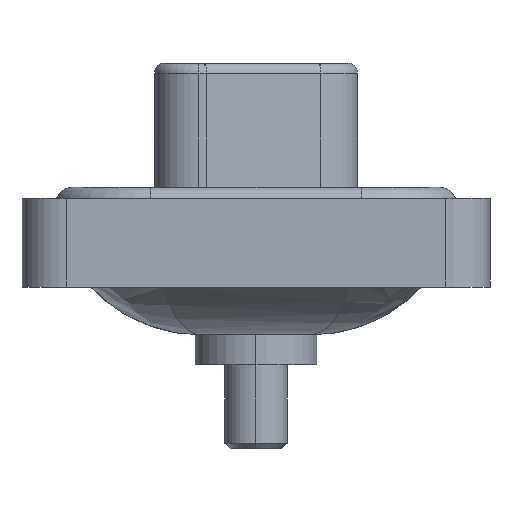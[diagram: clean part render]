
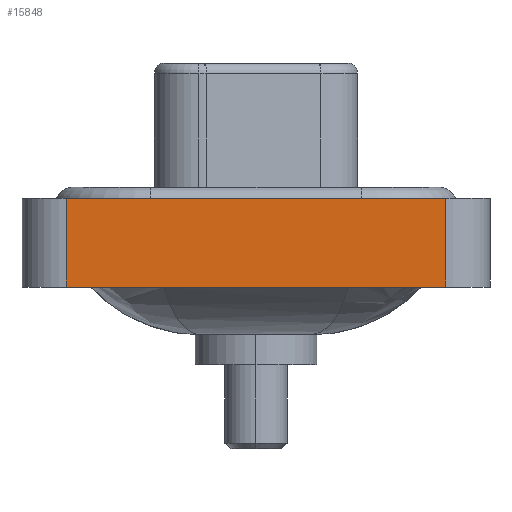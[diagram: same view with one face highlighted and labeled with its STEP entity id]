
A CAD part, left-side view. The second image highlights one B-rep face of the part: STEP entity #15848.
In plain terms, the highlighted planar face has unit normal (-1, 0, 0).
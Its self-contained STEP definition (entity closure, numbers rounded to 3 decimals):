
#290 = DIRECTION ( 'NONE',  ( 0., -1., 0. ) ) ;
#346 = EDGE_CURVE ( 'NONE', #10280, #13642, #2514, .T. ) ;
#699 = AXIS2_PLACEMENT_3D ( 'NONE', #17502, #13015, #10455 ) ;
#923 = LINE ( 'NONE', #11961, #15310 ) ;
#2514 = LINE ( 'NONE', #13461, #6872 ) ;
#2565 = VERTEX_POINT ( 'NONE', #12889 ) ;
#3357 = FACE_OUTER_BOUND ( 'NONE', #13291, .T. ) ;
#3530 = PLANE ( 'NONE',  #699 ) ;
#3637 = EDGE_CURVE ( 'NONE', #2565, #10280, #4622, .T. ) ;
#4595 = DIRECTION ( 'NONE',  ( 0., 0., 1. ) ) ;
#4622 = LINE ( 'NONE', #14352, #15995 ) ;
#6872 = VECTOR ( 'NONE', #13548, 1000. ) ;
#7420 = ORIENTED_EDGE ( 'NONE', *, *, #3637, .T. ) ;
#7435 = EDGE_CURVE ( 'NONE', #2565, #16762, #9113, .T. ) ;
#7573 = VECTOR ( 'NONE', #4595, 1000. ) ;
#8487 = ORIENTED_EDGE ( 'NONE', *, *, #7435, .F. ) ;
#8588 = ORIENTED_EDGE ( 'NONE', *, *, #9075, .F. ) ;
#9075 = EDGE_CURVE ( 'NONE', #16762, #13642, #923, .T. ) ;
#9087 = ORIENTED_EDGE ( 'NONE', *, *, #346, .T. ) ;
#9113 = LINE ( 'NONE', #14413, #7573 ) ;
#10280 = VERTEX_POINT ( 'NONE', #12982 ) ;
#10455 = DIRECTION ( 'NONE',  ( 0., 0., 1. ) ) ;
#11961 = CARTESIAN_POINT ( 'NONE',  ( -7.35, -8.55, 0.4 ) ) ;
#12889 = CARTESIAN_POINT ( 'NONE',  ( -7.35, 8.55, -3.6 ) ) ;
#12982 = CARTESIAN_POINT ( 'NONE',  ( -7.35, -8.55, -3.6 ) ) ;
#13015 = DIRECTION ( 'NONE',  ( -1., 0., 0. ) ) ;
#13291 = EDGE_LOOP ( 'NONE', ( #9087, #8588, #8487, #7420 ) ) ;
#13326 = CARTESIAN_POINT ( 'NONE',  ( -7.35, 8.55, 0.4 ) ) ;
#13461 = CARTESIAN_POINT ( 'NONE',  ( -7.35, -8.55, -3.6 ) ) ;
#13548 = DIRECTION ( 'NONE',  ( 0., 0., 1. ) ) ;
#13642 = VERTEX_POINT ( 'NONE', #14191 ) ;
#14191 = CARTESIAN_POINT ( 'NONE',  ( -7.35, -8.55, 0.4 ) ) ;
#14352 = CARTESIAN_POINT ( 'NONE',  ( -7.35, -8.55, -3.6 ) ) ;
#14413 = CARTESIAN_POINT ( 'NONE',  ( -7.35, 8.55, -3.6 ) ) ;
#14891 = DIRECTION ( 'NONE',  ( 0., -1., 0. ) ) ;
#15310 = VECTOR ( 'NONE', #14891, 1000. ) ;
#15848 = ADVANCED_FACE ( 'NONE', ( #3357 ), #3530, .T. ) ;
#15995 = VECTOR ( 'NONE', #290, 1000. ) ;
#16762 = VERTEX_POINT ( 'NONE', #13326 ) ;
#17502 = CARTESIAN_POINT ( 'NONE',  ( -7.35, -8.55, -3.6 ) ) ;
